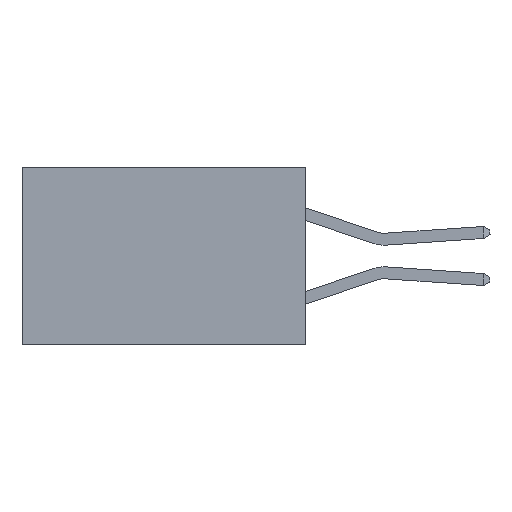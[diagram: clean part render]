
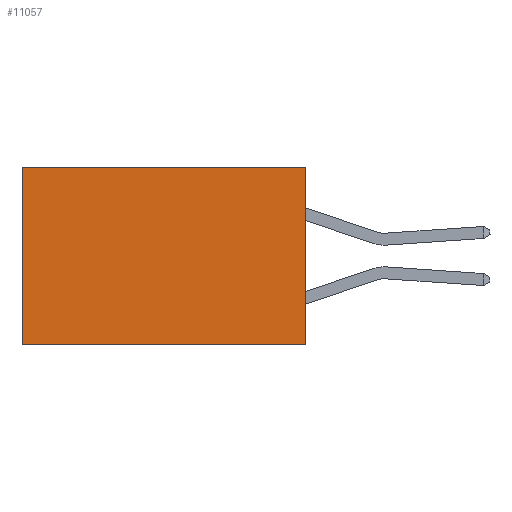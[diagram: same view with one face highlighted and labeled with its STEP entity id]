
A CAD part, left-side view. The second image highlights one B-rep face of the part: STEP entity #11057.
In plain terms, the highlighted planar face has unit normal (-1, 0, 0).
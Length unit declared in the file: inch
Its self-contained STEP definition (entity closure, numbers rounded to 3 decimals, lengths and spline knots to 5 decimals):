
#541 = EDGE_CURVE ( 'NONE', #9099, #2139, #4411, .T. ) ;
#729 = LINE ( 'NONE', #2145, #10609 ) ;
#1409 = VERTEX_POINT ( 'NONE', #7731 ) ;
#2139 = VERTEX_POINT ( 'NONE', #11331 ) ;
#2145 = CARTESIAN_POINT ( 'NONE',  ( 0.277, 0., -0.37 ) ) ;
#2527 = PLANE ( 'NONE',  #2956 ) ;
#2685 = DIRECTION ( 'NONE',  ( 0., 1., 0. ) ) ;
#2723 = EDGE_LOOP ( 'NONE', ( #11997, #10524, #11103, #4189 ) ) ;
#2956 = AXIS2_PLACEMENT_3D ( 'NONE', #9211, #10161, #4518 ) ;
#3097 = DIRECTION ( 'NONE',  ( 0., 0., -1. ) ) ;
#4165 = EDGE_CURVE ( 'NONE', #1409, #9099, #729, .T. ) ;
#4189 = ORIENTED_EDGE ( 'NONE', *, *, #4981, .T. ) ;
#4305 = DIRECTION ( 'NONE',  ( 0., 0., -1. ) ) ;
#4411 = LINE ( 'NONE', #8422, #9134 ) ;
#4518 = DIRECTION ( 'NONE',  ( 0., 0., -1. ) ) ;
#4928 = VECTOR ( 'NONE', #3097, 39.37008 ) ;
#4981 = EDGE_CURVE ( 'NONE', #1409, #7462, #6939, .T. ) ;
#5115 = CARTESIAN_POINT ( 'NONE',  ( 0.277, 0.59, 0. ) ) ;
#5734 = CARTESIAN_POINT ( 'NONE',  ( 0.277, 0., -0.37 ) ) ;
#6639 = VECTOR ( 'NONE', #6943, 39.37008 ) ;
#6855 = CARTESIAN_POINT ( 'NONE',  ( 0.277, 0., 0. ) ) ;
#6939 = LINE ( 'NONE', #6855, #6639 ) ;
#6943 = DIRECTION ( 'NONE',  ( 0., 1., 0. ) ) ;
#7158 = LINE ( 'NONE', #8811, #4928 ) ;
#7462 = VERTEX_POINT ( 'NONE', #5115 ) ;
#7731 = CARTESIAN_POINT ( 'NONE',  ( 0.277, 0., 0. ) ) ;
#8044 = EDGE_CURVE ( 'NONE', #7462, #2139, #7158, .T. ) ;
#8422 = CARTESIAN_POINT ( 'NONE',  ( 0.277, 0., -0.37 ) ) ;
#8811 = CARTESIAN_POINT ( 'NONE',  ( 0.277, 0.59, -0.37 ) ) ;
#9099 = VERTEX_POINT ( 'NONE', #5734 ) ;
#9134 = VECTOR ( 'NONE', #2685, 39.37008 ) ;
#9165 = FACE_OUTER_BOUND ( 'NONE', #2723, .T. ) ;
#9211 = CARTESIAN_POINT ( 'NONE',  ( 0.277, 0., -0.37 ) ) ;
#10161 = DIRECTION ( 'NONE',  ( 1., 0., 0. ) ) ;
#10524 = ORIENTED_EDGE ( 'NONE', *, *, #541, .F. ) ;
#10609 = VECTOR ( 'NONE', #4305, 39.37008 ) ;
#11057 = ADVANCED_FACE ( 'NONE', ( #9165 ), #2527, .F. ) ;
#11103 = ORIENTED_EDGE ( 'NONE', *, *, #4165, .F. ) ;
#11331 = CARTESIAN_POINT ( 'NONE',  ( 0.277, 0.59, -0.37 ) ) ;
#11997 = ORIENTED_EDGE ( 'NONE', *, *, #8044, .T. ) ;
